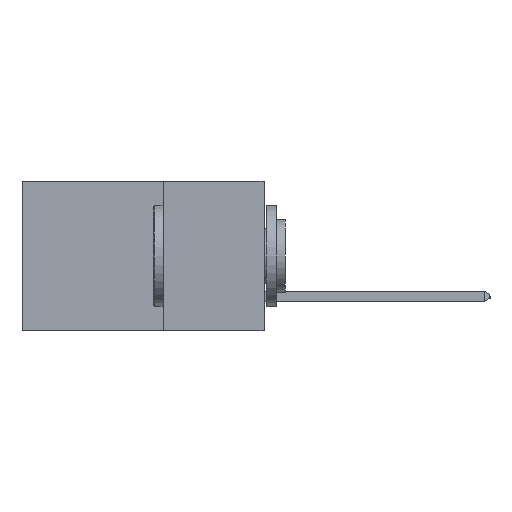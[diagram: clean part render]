
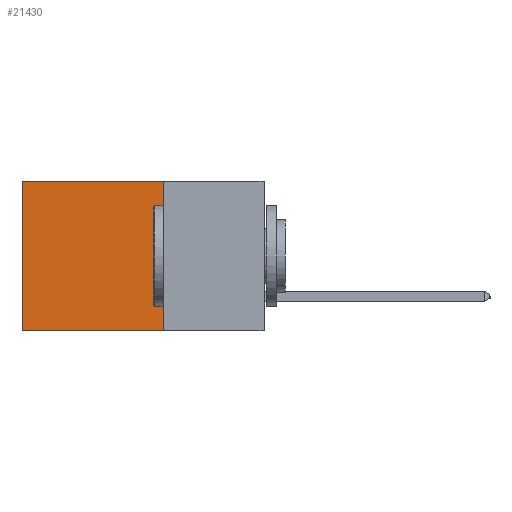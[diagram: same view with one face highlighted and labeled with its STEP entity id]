
A CAD part, left-side view. The second image highlights one B-rep face of the part: STEP entity #21430.
In plain terms, the highlighted planar face has unit normal (-1, 0, 0).
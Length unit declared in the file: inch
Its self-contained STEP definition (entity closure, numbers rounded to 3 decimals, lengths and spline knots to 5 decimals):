
#275 = VECTOR ( 'NONE', #20150, 39.37008 ) ;
#722 = ORIENTED_EDGE ( 'NONE', *, *, #864, .T. ) ;
#864 = EDGE_CURVE ( 'NONE', #21453, #1114, #21304, .T. ) ;
#936 = DIRECTION ( 'NONE',  ( 1., 0., 0. ) ) ;
#1114 = VERTEX_POINT ( 'NONE', #16286 ) ;
#1286 = CARTESIAN_POINT ( 'NONE',  ( 0.298, 0.25, 0. ) ) ;
#1508 = CARTESIAN_POINT ( 'NONE',  ( 0.298, 0.25, 0. ) ) ;
#2647 = LINE ( 'NONE', #26560, #23577 ) ;
#2710 = ORIENTED_EDGE ( 'NONE', *, *, #19937, .T. ) ;
#3546 = AXIS2_PLACEMENT_3D ( 'NONE', #21781, #936, #15632 ) ;
#5280 = EDGE_LOOP ( 'NONE', ( #722, #23812, #7033, #2710 ) ) ;
#6417 = LINE ( 'NONE', #1286, #275 ) ;
#7033 = ORIENTED_EDGE ( 'NONE', *, *, #12101, .F. ) ;
#8922 = CARTESIAN_POINT ( 'NONE',  ( 0.298, 0.25, -0.37 ) ) ;
#9467 = VECTOR ( 'NONE', #23945, 39.37008 ) ;
#12101 = EDGE_CURVE ( 'NONE', #15148, #19081, #2647, .T. ) ;
#12944 = VECTOR ( 'NONE', #25663, 39.37008 ) ;
#15106 = CARTESIAN_POINT ( 'NONE',  ( 0.298, 0.25, -0.37 ) ) ;
#15148 = VERTEX_POINT ( 'NONE', #1508 ) ;
#15632 = DIRECTION ( 'NONE',  ( 0., 0., -1. ) ) ;
#15945 = FACE_OUTER_BOUND ( 'NONE', #5280, .T. ) ;
#16286 = CARTESIAN_POINT ( 'NONE',  ( 0.298, 0.6, -0.37 ) ) ;
#17059 = CARTESIAN_POINT ( 'NONE',  ( 0.298, 0.6, 0. ) ) ;
#17750 = CARTESIAN_POINT ( 'NONE',  ( 0.298, 0.6, 0. ) ) ;
#19081 = VERTEX_POINT ( 'NONE', #15106 ) ;
#19937 = EDGE_CURVE ( 'NONE', #15148, #21453, #6417, .T. ) ;
#20150 = DIRECTION ( 'NONE',  ( 0., 1., 0. ) ) ;
#21304 = LINE ( 'NONE', #17059, #9467 ) ;
#21430 = ADVANCED_FACE ( 'NONE', ( #15945 ), #25900, .F. ) ;
#21453 = VERTEX_POINT ( 'NONE', #17750 ) ;
#21781 = CARTESIAN_POINT ( 'NONE',  ( 0.298, 0.25, 0. ) ) ;
#22543 = DIRECTION ( 'NONE',  ( 0., 0., -1. ) ) ;
#23577 = VECTOR ( 'NONE', #22543, 39.37008 ) ;
#23812 = ORIENTED_EDGE ( 'NONE', *, *, #26449, .F. ) ;
#23945 = DIRECTION ( 'NONE',  ( 0., 0., -1. ) ) ;
#23984 = LINE ( 'NONE', #8922, #12944 ) ;
#25663 = DIRECTION ( 'NONE',  ( 0., 1., 0. ) ) ;
#25900 = PLANE ( 'NONE',  #3546 ) ;
#26449 = EDGE_CURVE ( 'NONE', #19081, #1114, #23984, .T. ) ;
#26560 = CARTESIAN_POINT ( 'NONE',  ( 0.298, 0.25, 0. ) ) ;
